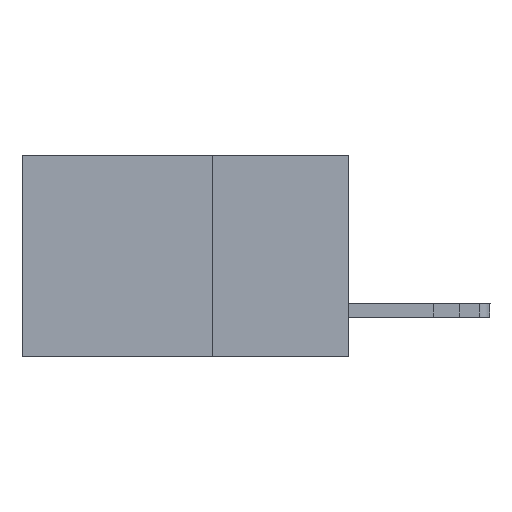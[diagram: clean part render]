
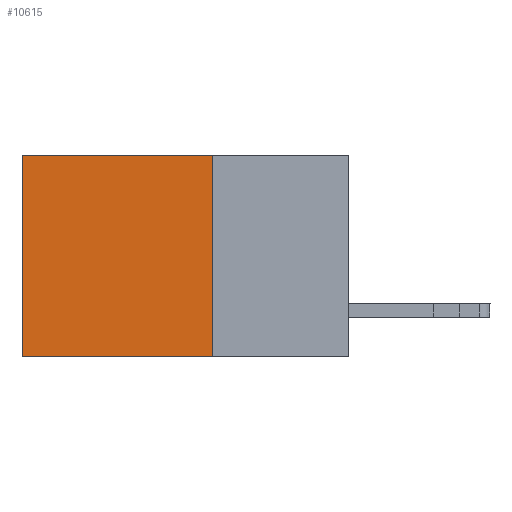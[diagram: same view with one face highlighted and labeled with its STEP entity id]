
A CAD part, left-side view. The second image highlights one B-rep face of the part: STEP entity #10615.
In plain terms, the highlighted planar face has unit normal (-1, 0, 0).
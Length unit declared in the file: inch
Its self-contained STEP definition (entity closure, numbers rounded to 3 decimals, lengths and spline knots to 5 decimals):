
#42 = VECTOR ( 'NONE', #9510, 39.37008 ) ;
#354 = DIRECTION ( 'NONE',  ( 0., 0., -1. ) ) ;
#557 = DIRECTION ( 'NONE',  ( 0., 1., 0. ) ) ;
#1829 = DIRECTION ( 'NONE',  ( 0., 1., 0. ) ) ;
#1830 = AXIS2_PLACEMENT_3D ( 'NONE', #9257, #4838, #354 ) ;
#2074 = FACE_OUTER_BOUND ( 'NONE', #7416, .T. ) ;
#2359 = VERTEX_POINT ( 'NONE', #2568 ) ;
#2374 = LINE ( 'NONE', #4964, #42 ) ;
#2568 = CARTESIAN_POINT ( 'NONE',  ( 0.2615, 0.6, -0.37 ) ) ;
#3435 = LINE ( 'NONE', #11435, #3534 ) ;
#3467 = ORIENTED_EDGE ( 'NONE', *, *, #5810, .T. ) ;
#3534 = VECTOR ( 'NONE', #557, 39.37008 ) ;
#3559 = LINE ( 'NONE', #7078, #6255 ) ;
#3891 = VERTEX_POINT ( 'NONE', #6449 ) ;
#4647 = EDGE_CURVE ( 'NONE', #9682, #9876, #5358, .T. ) ;
#4744 = ORIENTED_EDGE ( 'NONE', *, *, #11193, .F. ) ;
#4838 = DIRECTION ( 'NONE',  ( 1., 0., 0. ) ) ;
#4964 = CARTESIAN_POINT ( 'NONE',  ( 0.2615, 0.6, -0.37 ) ) ;
#5358 = LINE ( 'NONE', #9789, #10025 ) ;
#5489 = DIRECTION ( 'NONE',  ( 0., 0., -1. ) ) ;
#5490 = ORIENTED_EDGE ( 'NONE', *, *, #4647, .T. ) ;
#5594 = EDGE_CURVE ( 'NONE', #9682, #3891, #3559, .T. ) ;
#5773 = PLANE ( 'NONE',  #1830 ) ;
#5810 = EDGE_CURVE ( 'NONE', #9876, #2359, #2374, .T. ) ;
#6255 = VECTOR ( 'NONE', #5489, 39.37008 ) ;
#6449 = CARTESIAN_POINT ( 'NONE',  ( 0.2615, 0.25, -0.37 ) ) ;
#7078 = CARTESIAN_POINT ( 'NONE',  ( 0.2615, 0.25, -0.37 ) ) ;
#7416 = EDGE_LOOP ( 'NONE', ( #3467, #4744, #8612, #5490 ) ) ;
#8612 = ORIENTED_EDGE ( 'NONE', *, *, #5594, .F. ) ;
#9257 = CARTESIAN_POINT ( 'NONE',  ( 0.2615, 0.25, -0.37 ) ) ;
#9510 = DIRECTION ( 'NONE',  ( 0., 0., -1. ) ) ;
#9682 = VERTEX_POINT ( 'NONE', #10934 ) ;
#9789 = CARTESIAN_POINT ( 'NONE',  ( 0.2615, 0.25, 0. ) ) ;
#9876 = VERTEX_POINT ( 'NONE', #10404 ) ;
#10025 = VECTOR ( 'NONE', #1829, 39.37008 ) ;
#10404 = CARTESIAN_POINT ( 'NONE',  ( 0.2615, 0.6, 0. ) ) ;
#10615 = ADVANCED_FACE ( 'NONE', ( #2074 ), #5773, .F. ) ;
#10934 = CARTESIAN_POINT ( 'NONE',  ( 0.2615, 0.25, 0. ) ) ;
#11193 = EDGE_CURVE ( 'NONE', #3891, #2359, #3435, .T. ) ;
#11435 = CARTESIAN_POINT ( 'NONE',  ( 0.2615, 0.25, -0.37 ) ) ;
